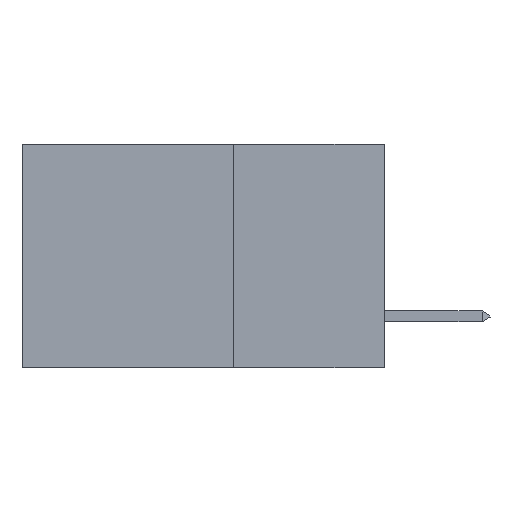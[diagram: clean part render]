
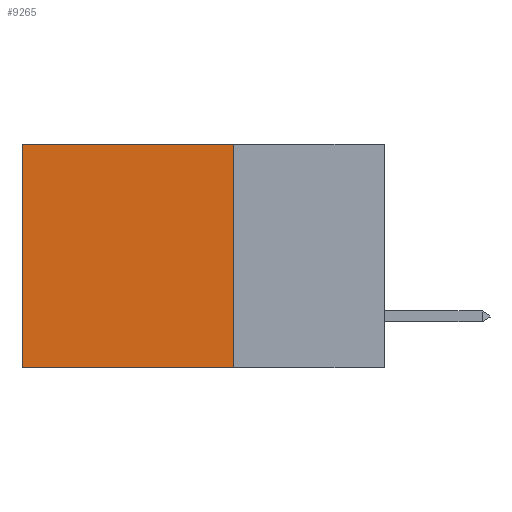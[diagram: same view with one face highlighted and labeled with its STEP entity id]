
A CAD part, left-side view. The second image highlights one B-rep face of the part: STEP entity #9265.
In plain terms, the highlighted planar face has unit normal (-1, 0, 0).
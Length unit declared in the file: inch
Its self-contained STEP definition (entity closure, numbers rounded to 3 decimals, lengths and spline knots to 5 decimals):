
#1014 = DIRECTION ( 'NONE',  ( 0., 0., -1. ) ) ;
#2216 = LINE ( 'NONE', #7067, #27958 ) ;
#3742 = CARTESIAN_POINT ( 'NONE',  ( 0.2875, 0.6, 0. ) ) ;
#5322 = VECTOR ( 'NONE', #23759, 39.37008 ) ;
#6202 = CARTESIAN_POINT ( 'NONE',  ( 0.2875, 0.25, 0. ) ) ;
#7067 = CARTESIAN_POINT ( 'NONE',  ( 0.2875, 0.25, -0.37 ) ) ;
#9265 = ADVANCED_FACE ( 'NONE', ( #31156 ), #27933, .F. ) ;
#9528 = DIRECTION ( 'NONE',  ( 0., 0., -1. ) ) ;
#9722 = VERTEX_POINT ( 'NONE', #12705 ) ;
#10902 = DIRECTION ( 'NONE',  ( 1., 0., 0. ) ) ;
#11505 = CARTESIAN_POINT ( 'NONE',  ( 0.2875, 0.25, 0. ) ) ;
#12705 = CARTESIAN_POINT ( 'NONE',  ( 0.2875, 0.25, -0.37 ) ) ;
#13258 = CARTESIAN_POINT ( 'NONE',  ( 0.2875, 0.6, -0.37 ) ) ;
#13759 = ORIENTED_EDGE ( 'NONE', *, *, #30548, .T. ) ;
#13982 = EDGE_LOOP ( 'NONE', ( #13759, #25668, #30833, #30139 ) ) ;
#14714 = LINE ( 'NONE', #11505, #5322 ) ;
#15332 = LINE ( 'NONE', #24489, #26747 ) ;
#16456 = AXIS2_PLACEMENT_3D ( 'NONE', #6202, #10902, #1014 ) ;
#17426 = CARTESIAN_POINT ( 'NONE',  ( 0.2875, 0.6, 0. ) ) ;
#19064 = LINE ( 'NONE', #17426, #26913 ) ;
#19972 = VERTEX_POINT ( 'NONE', #3742 ) ;
#20140 = DIRECTION ( 'NONE',  ( 0., 1., 0. ) ) ;
#20611 = EDGE_CURVE ( 'NONE', #22450, #19972, #14714, .T. ) ;
#22450 = VERTEX_POINT ( 'NONE', #29415 ) ;
#23759 = DIRECTION ( 'NONE',  ( 0., 1., 0. ) ) ;
#24489 = CARTESIAN_POINT ( 'NONE',  ( 0.2875, 0.25, 0. ) ) ;
#24902 = EDGE_CURVE ( 'NONE', #9722, #25045, #2216, .T. ) ;
#25045 = VERTEX_POINT ( 'NONE', #13258 ) ;
#25668 = ORIENTED_EDGE ( 'NONE', *, *, #24902, .F. ) ;
#26620 = EDGE_CURVE ( 'NONE', #22450, #9722, #15332, .T. ) ;
#26747 = VECTOR ( 'NONE', #9528, 39.37008 ) ;
#26913 = VECTOR ( 'NONE', #29688, 39.37008 ) ;
#27933 = PLANE ( 'NONE',  #16456 ) ;
#27958 = VECTOR ( 'NONE', #20140, 39.37008 ) ;
#29415 = CARTESIAN_POINT ( 'NONE',  ( 0.2875, 0.25, 0. ) ) ;
#29688 = DIRECTION ( 'NONE',  ( 0., 0., -1. ) ) ;
#30139 = ORIENTED_EDGE ( 'NONE', *, *, #20611, .T. ) ;
#30548 = EDGE_CURVE ( 'NONE', #19972, #25045, #19064, .T. ) ;
#30833 = ORIENTED_EDGE ( 'NONE', *, *, #26620, .F. ) ;
#31156 = FACE_OUTER_BOUND ( 'NONE', #13982, .T. ) ;
